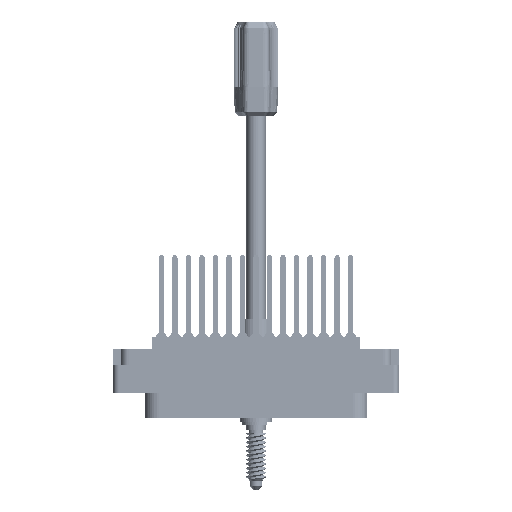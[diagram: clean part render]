
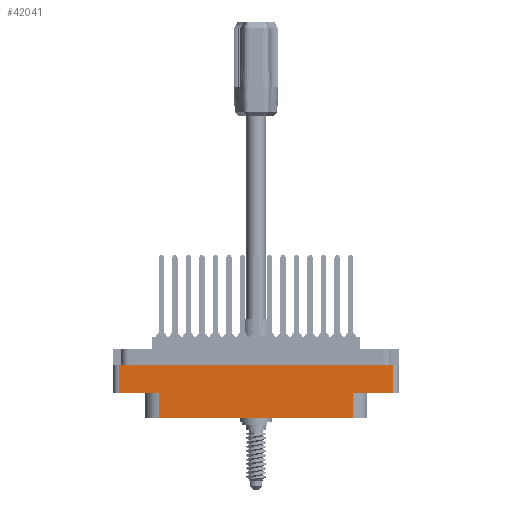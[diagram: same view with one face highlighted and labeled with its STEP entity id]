
A CAD part, front view. The second image highlights one B-rep face of the part: STEP entity #42041.
In plain terms, the highlighted planar face has unit normal (0, -1, 0).
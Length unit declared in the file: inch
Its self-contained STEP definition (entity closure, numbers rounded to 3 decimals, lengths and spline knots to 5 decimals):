
#1576 = PLANE ( 'NONE',  #25410 ) ;
#2765 = LINE ( 'NONE', #28046, #40175 ) ;
#3956 = DIRECTION ( 'NONE',  ( 1., 0., 0. ) ) ;
#4353 = DIRECTION ( 'NONE',  ( -1., 0., 0. ) ) ;
#5281 = VERTEX_POINT ( 'NONE', #94729 ) ;
#5290 = VERTEX_POINT ( 'NONE', #71685 ) ;
#5784 = CARTESIAN_POINT ( 'NONE',  ( 0.9315, -0.7625, -0.54 ) ) ;
#6526 = VECTOR ( 'NONE', #4353, 39.37008 ) ;
#7058 = ORIENTED_EDGE ( 'NONE', *, *, #99064, .T. ) ;
#7743 = CARTESIAN_POINT ( 'NONE',  ( -0.9315, -0.7625, -0.78 ) ) ;
#12312 = DIRECTION ( 'NONE',  ( 0., 0., 1. ) ) ;
#13481 = LINE ( 'NONE', #13789, #52245 ) ;
#13789 = CARTESIAN_POINT ( 'NONE',  ( -1.313, -0.7625, -0.78 ) ) ;
#14939 = FACE_OUTER_BOUND ( 'NONE', #58047, .T. ) ;
#18089 = VECTOR ( 'NONE', #12312, 39.37008 ) ;
#18300 = CARTESIAN_POINT ( 'NONE',  ( 0.9315, -0.7625, -0.78 ) ) ;
#19216 = EDGE_CURVE ( 'NONE', #29624, #78981, #74078, .T. ) ;
#21024 = VERTEX_POINT ( 'NONE', #41148 ) ;
#24231 = ORIENTED_EDGE ( 'NONE', *, *, #66684, .T. ) ;
#24271 = CARTESIAN_POINT ( 'NONE',  ( -1.375, -0.7625, -0.78 ) ) ;
#25410 = AXIS2_PLACEMENT_3D ( 'NONE', #24271, #56380, #73116 ) ;
#25592 = LINE ( 'NONE', #67784, #18089 ) ;
#28046 = CARTESIAN_POINT ( 'NONE',  ( 0., -0.7625, -0.54 ) ) ;
#29624 = VERTEX_POINT ( 'NONE', #66285 ) ;
#29742 = VERTEX_POINT ( 'NONE', #18300 ) ;
#32256 = CARTESIAN_POINT ( 'NONE',  ( -1.313, -0.7625, -0.54 ) ) ;
#34074 = VERTEX_POINT ( 'NONE', #32256 ) ;
#36555 = EDGE_CURVE ( 'NONE', #93318, #29742, #44400, .T. ) ;
#37482 = LINE ( 'NONE', #73826, #43678 ) ;
#40175 = VECTOR ( 'NONE', #3956, 39.37008 ) ;
#40677 = VECTOR ( 'NONE', #63254, 39.37008 ) ;
#41148 = CARTESIAN_POINT ( 'NONE',  ( -0.9315, -0.7625, -0.54 ) ) ;
#42041 = ADVANCED_FACE ( 'NONE', ( #14939 ), #1576, .T. ) ;
#42160 = ORIENTED_EDGE ( 'NONE', *, *, #46225, .T. ) ;
#42259 = CARTESIAN_POINT ( 'NONE',  ( 0., -0.7625, -0.274 ) ) ;
#42619 = VECTOR ( 'NONE', #90414, 39.37008 ) ;
#43678 = VECTOR ( 'NONE', #88452, 39.37008 ) ;
#43785 = CARTESIAN_POINT ( 'NONE',  ( 0., -0.7625, -0.54 ) ) ;
#44400 = LINE ( 'NONE', #62549, #40677 ) ;
#46225 = EDGE_CURVE ( 'NONE', #34074, #21024, #2765, .T. ) ;
#49491 = ORIENTED_EDGE ( 'NONE', *, *, #90928, .T. ) ;
#52208 = DIRECTION ( 'NONE',  ( 0., 0., 1. ) ) ;
#52245 = VECTOR ( 'NONE', #60599, 39.37008 ) ;
#56228 = ORIENTED_EDGE ( 'NONE', *, *, #98945, .T. ) ;
#56380 = DIRECTION ( 'NONE',  ( 0., -1., 0. ) ) ;
#58047 = EDGE_LOOP ( 'NONE', ( #97434, #7058, #42160, #49491, #73216, #24231, #99453, #56228 ) ) ;
#60599 = DIRECTION ( 'NONE',  ( 0., 0., -1. ) ) ;
#62549 = CARTESIAN_POINT ( 'NONE',  ( -1.375, -0.7625, -0.78 ) ) ;
#63254 = DIRECTION ( 'NONE',  ( 1., 0., 0. ) ) ;
#63449 = VECTOR ( 'NONE', #52208, 39.37008 ) ;
#66285 = CARTESIAN_POINT ( 'NONE',  ( 1.313, -0.7625, -0.54 ) ) ;
#66684 = EDGE_CURVE ( 'NONE', #29742, #78981, #25592, .T. ) ;
#66898 = CARTESIAN_POINT ( 'NONE',  ( 1.313, -0.7625, -0.78 ) ) ;
#67784 = CARTESIAN_POINT ( 'NONE',  ( 0.9315, -0.7625, -0.54 ) ) ;
#71303 = EDGE_CURVE ( 'NONE', #5290, #5281, #71355, .T. ) ;
#71355 = LINE ( 'NONE', #42259, #42619 ) ;
#71685 = CARTESIAN_POINT ( 'NONE',  ( -1.313, -0.7625, -0.274 ) ) ;
#73116 = DIRECTION ( 'NONE',  ( 0., 0., -1. ) ) ;
#73216 = ORIENTED_EDGE ( 'NONE', *, *, #36555, .T. ) ;
#73826 = CARTESIAN_POINT ( 'NONE',  ( -0.9315, -0.7625, -0.78 ) ) ;
#74078 = LINE ( 'NONE', #43785, #6526 ) ;
#78981 = VERTEX_POINT ( 'NONE', #5784 ) ;
#82169 = LINE ( 'NONE', #66898, #63449 ) ;
#88452 = DIRECTION ( 'NONE',  ( 0., 0., -1. ) ) ;
#90414 = DIRECTION ( 'NONE',  ( 1., 0., 0. ) ) ;
#90928 = EDGE_CURVE ( 'NONE', #21024, #93318, #37482, .T. ) ;
#93318 = VERTEX_POINT ( 'NONE', #7743 ) ;
#94729 = CARTESIAN_POINT ( 'NONE',  ( 1.313, -0.7625, -0.274 ) ) ;
#97434 = ORIENTED_EDGE ( 'NONE', *, *, #71303, .F. ) ;
#98945 = EDGE_CURVE ( 'NONE', #29624, #5281, #82169, .T. ) ;
#99064 = EDGE_CURVE ( 'NONE', #5290, #34074, #13481, .T. ) ;
#99453 = ORIENTED_EDGE ( 'NONE', *, *, #19216, .F. ) ;
